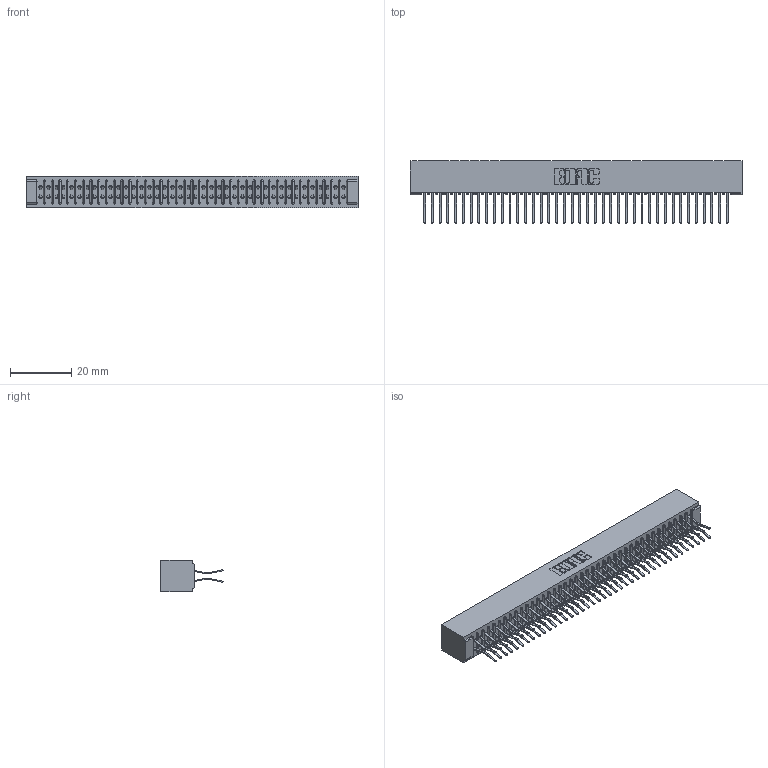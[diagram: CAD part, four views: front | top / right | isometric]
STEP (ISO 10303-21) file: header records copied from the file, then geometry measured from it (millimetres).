
FILE_DESCRIPTION (( 'STEP AP203' ), '1' );
FILE_NAME ('391-080-560-201.STEP', '2018-08-09T15:48:54', ( '' ), ( '' ), 'SwSTEP 2.0', 'SolidWorks 2016', '' );
FILE_SCHEMA (( 'CONFIG_CONTROL_DESIGN' ));
Length unit declared in the file: inch
Products named in the file (3): 341 Part_No Mounting Lugs; 341-292-001_341-292-160; 391-080-560-201
Assembly tree (81 placements, depth 2):
  391-080-560-201
    341 Part_No Mounting Lugs
    341-292-001_341-292-160  x80
Bounding box: 108.58 x 20.37 x 10.16 mm (x, y, z)
Volume: 8332 mm3; surface area: 15981.6 mm2
Topology: 81 solids, 81 shells, 5708 faces, 16572 edges, 10750 vertices
Faces by surface type: plane 3264, cylinder 2284, sphere 82, torus 78
Entity records: 48537 total; most frequent: CARTESIAN_POINT 8068, ORIENTED_EDGE 8016, DIRECTION 7834, EDGE_CURVE 4008, VECTOR 3234, LINE 3234, VERTEX_POINT 2534, AXIS2_PLACEMENT_3D 2300
